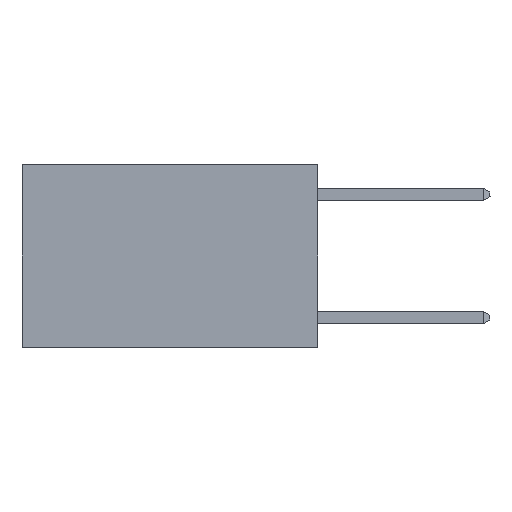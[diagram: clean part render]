
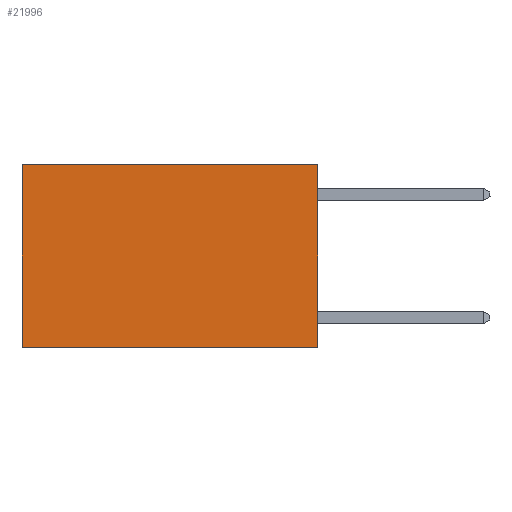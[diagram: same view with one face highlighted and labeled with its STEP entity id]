
A CAD part, left-side view. The second image highlights one B-rep face of the part: STEP entity #21996.
In plain terms, the highlighted planar face has unit normal (-1, 0, 0).
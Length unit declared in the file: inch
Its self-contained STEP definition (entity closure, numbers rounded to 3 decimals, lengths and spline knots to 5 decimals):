
#386 = ORIENTED_EDGE ( 'NONE', *, *, #17037, .T. ) ;
#1142 = VERTEX_POINT ( 'NONE', #17708 ) ;
#2242 = VERTEX_POINT ( 'NONE', #2540 ) ;
#2540 = CARTESIAN_POINT ( 'NONE',  ( 0.2625, 0.6, 0. ) ) ;
#4380 = EDGE_LOOP ( 'NONE', ( #386, #16168, #8612, #25157 ) ) ;
#4671 = CARTESIAN_POINT ( 'NONE',  ( 0.2625, 0.6, 0. ) ) ;
#5576 = PLANE ( 'NONE',  #19823 ) ;
#6114 = DIRECTION ( 'NONE',  ( 0., 1., 0. ) ) ;
#6456 = CARTESIAN_POINT ( 'NONE',  ( 0.2625, 0., 0. ) ) ;
#8612 = ORIENTED_EDGE ( 'NONE', *, *, #17584, .F. ) ;
#9456 = EDGE_CURVE ( 'NONE', #11477, #10358, #18515, .T. ) ;
#10334 = DIRECTION ( 'NONE',  ( 0., 1., 0. ) ) ;
#10358 = VERTEX_POINT ( 'NONE', #25460 ) ;
#10424 = CARTESIAN_POINT ( 'NONE',  ( 0.2625, 0., -0.37 ) ) ;
#10507 = VECTOR ( 'NONE', #10334, 39.37008 ) ;
#11477 = VERTEX_POINT ( 'NONE', #18217 ) ;
#12219 = DIRECTION ( 'NONE',  ( 0., 0., -1. ) ) ;
#13153 = DIRECTION ( 'NONE',  ( 0., 0., -1. ) ) ;
#13417 = CARTESIAN_POINT ( 'NONE',  ( 0.2625, 0., 0. ) ) ;
#14141 = EDGE_CURVE ( 'NONE', #1142, #2242, #19296, .T. ) ;
#15482 = VECTOR ( 'NONE', #16165, 39.37008 ) ;
#15779 = LINE ( 'NONE', #4671, #15482 ) ;
#16165 = DIRECTION ( 'NONE',  ( 0., 0., -1. ) ) ;
#16168 = ORIENTED_EDGE ( 'NONE', *, *, #9456, .F. ) ;
#16557 = FACE_OUTER_BOUND ( 'NONE', #4380, .T. ) ;
#17037 = EDGE_CURVE ( 'NONE', #2242, #10358, #15779, .T. ) ;
#17584 = EDGE_CURVE ( 'NONE', #1142, #11477, #23840, .T. ) ;
#17708 = CARTESIAN_POINT ( 'NONE',  ( 0.2625, 0., 0. ) ) ;
#18217 = CARTESIAN_POINT ( 'NONE',  ( 0.2625, 0., -0.37 ) ) ;
#18515 = LINE ( 'NONE', #10424, #10507 ) ;
#18522 = VECTOR ( 'NONE', #13153, 39.37008 ) ;
#19296 = LINE ( 'NONE', #19643, #25203 ) ;
#19643 = CARTESIAN_POINT ( 'NONE',  ( 0.2625, 0., 0. ) ) ;
#19823 = AXIS2_PLACEMENT_3D ( 'NONE', #6456, #19976, #12219 ) ;
#19976 = DIRECTION ( 'NONE',  ( 1., 0., 0. ) ) ;
#21996 = ADVANCED_FACE ( 'NONE', ( #16557 ), #5576, .F. ) ;
#23840 = LINE ( 'NONE', #13417, #18522 ) ;
#25157 = ORIENTED_EDGE ( 'NONE', *, *, #14141, .T. ) ;
#25203 = VECTOR ( 'NONE', #6114, 39.37008 ) ;
#25460 = CARTESIAN_POINT ( 'NONE',  ( 0.2625, 0.6, -0.37 ) ) ;
